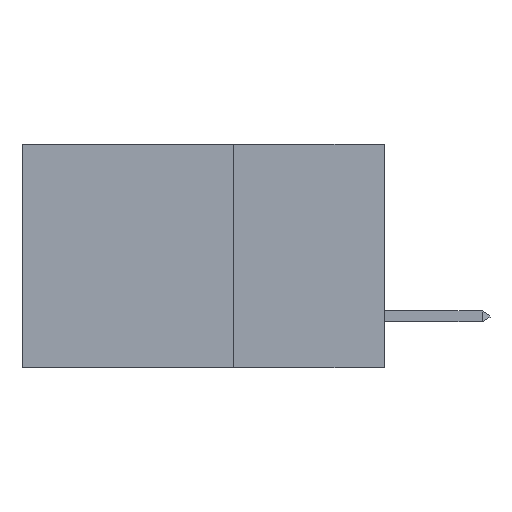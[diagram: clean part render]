
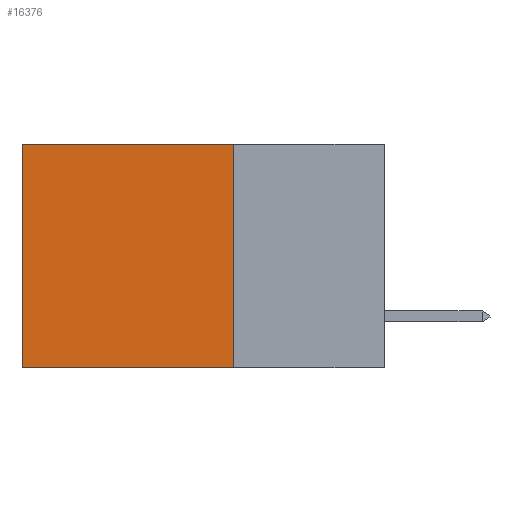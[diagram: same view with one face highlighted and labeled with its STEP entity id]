
A CAD part, left-side view. The second image highlights one B-rep face of the part: STEP entity #16376.
In plain terms, the highlighted planar face has unit normal (-1, 0, 0).
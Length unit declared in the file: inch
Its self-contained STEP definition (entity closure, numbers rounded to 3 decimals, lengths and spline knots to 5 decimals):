
#268 = ORIENTED_EDGE ( 'NONE', *, *, #6875, .F. ) ;
#377 = CARTESIAN_POINT ( 'NONE',  ( 0.2875, 0.25, 0. ) ) ;
#441 = LINE ( 'NONE', #9471, #7705 ) ;
#462 = CARTESIAN_POINT ( 'NONE',  ( 0.2875, 0.25, -0.37 ) ) ;
#671 = PLANE ( 'NONE',  #3769 ) ;
#711 = VERTEX_POINT ( 'NONE', #6454 ) ;
#889 = LINE ( 'NONE', #377, #4341 ) ;
#1745 = VERTEX_POINT ( 'NONE', #12595 ) ;
#2073 = CARTESIAN_POINT ( 'NONE',  ( 0.2875, 0.6, 0. ) ) ;
#2183 = VECTOR ( 'NONE', #10406, 39.37008 ) ;
#2203 = CARTESIAN_POINT ( 'NONE',  ( 0.2875, 0.25, 0. ) ) ;
#3271 = DIRECTION ( 'NONE',  ( 0., 1., 0. ) ) ;
#3396 = CARTESIAN_POINT ( 'NONE',  ( 0.2875, 0.6, 0. ) ) ;
#3769 = AXIS2_PLACEMENT_3D ( 'NONE', #2203, #6638, #16124 ) ;
#4341 = VECTOR ( 'NONE', #3271, 39.37008 ) ;
#5402 = ORIENTED_EDGE ( 'NONE', *, *, #15183, .F. ) ;
#6068 = CARTESIAN_POINT ( 'NONE',  ( 0.2875, 0.6, -0.37 ) ) ;
#6454 = CARTESIAN_POINT ( 'NONE',  ( 0.2875, 0.25, 0. ) ) ;
#6638 = DIRECTION ( 'NONE',  ( 1., 0., 0. ) ) ;
#6875 = EDGE_CURVE ( 'NONE', #1745, #8673, #12913, .T. ) ;
#7530 = EDGE_CURVE ( 'NONE', #16309, #8673, #12918, .T. ) ;
#7705 = VECTOR ( 'NONE', #12124, 39.37008 ) ;
#8673 = VERTEX_POINT ( 'NONE', #6068 ) ;
#8747 = FACE_OUTER_BOUND ( 'NONE', #11212, .T. ) ;
#9312 = VECTOR ( 'NONE', #15838, 39.37008 ) ;
#9471 = CARTESIAN_POINT ( 'NONE',  ( 0.2875, 0.25, 0. ) ) ;
#10406 = DIRECTION ( 'NONE',  ( 0., 1., 0. ) ) ;
#11212 = EDGE_LOOP ( 'NONE', ( #16577, #268, #5402, #13894 ) ) ;
#12124 = DIRECTION ( 'NONE',  ( 0., 0., -1. ) ) ;
#12595 = CARTESIAN_POINT ( 'NONE',  ( 0.2875, 0.25, -0.37 ) ) ;
#12913 = LINE ( 'NONE', #462, #2183 ) ;
#12918 = LINE ( 'NONE', #3396, #9312 ) ;
#13894 = ORIENTED_EDGE ( 'NONE', *, *, #15573, .T. ) ;
#15183 = EDGE_CURVE ( 'NONE', #711, #1745, #441, .T. ) ;
#15573 = EDGE_CURVE ( 'NONE', #711, #16309, #889, .T. ) ;
#15838 = DIRECTION ( 'NONE',  ( 0., 0., -1. ) ) ;
#16124 = DIRECTION ( 'NONE',  ( 0., 0., -1. ) ) ;
#16309 = VERTEX_POINT ( 'NONE', #2073 ) ;
#16376 = ADVANCED_FACE ( 'NONE', ( #8747 ), #671, .F. ) ;
#16577 = ORIENTED_EDGE ( 'NONE', *, *, #7530, .T. ) ;
